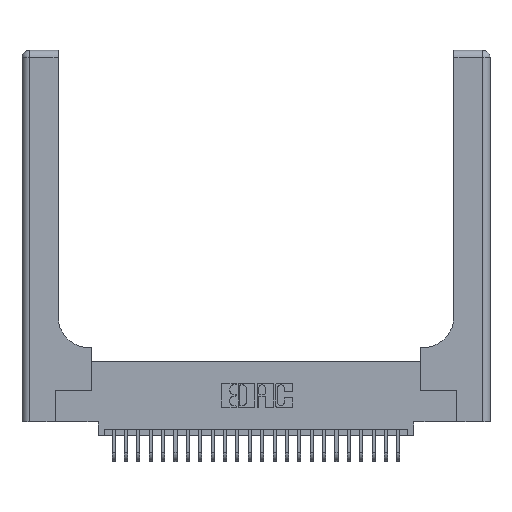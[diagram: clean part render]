
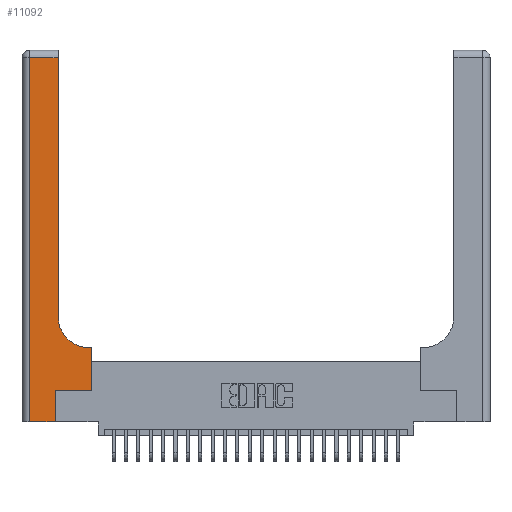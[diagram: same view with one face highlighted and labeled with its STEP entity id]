
A CAD part, top view. The second image highlights one B-rep face of the part: STEP entity #11092.
In plain terms, the highlighted planar face has unit normal (0, 0, 1).
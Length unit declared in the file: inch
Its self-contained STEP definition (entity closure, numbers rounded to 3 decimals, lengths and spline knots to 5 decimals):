
#36 = ORIENTED_EDGE ( 'NONE', *, *, #11155, .T. ) ;
#341 = VECTOR ( 'NONE', #14687, 39.37008 ) ;
#503 = CIRCLE ( 'NONE', #4987, 0.25 ) ;
#519 = EDGE_CURVE ( 'NONE', #6379, #22907, #762, .T. ) ;
#762 = LINE ( 'NONE', #20495, #17562 ) ;
#1103 = DIRECTION ( 'NONE',  ( -1., 0., 0. ) ) ;
#1154 = LINE ( 'NONE', #1720, #12187 ) ;
#1498 = DIRECTION ( 'NONE',  ( -1., 0., 0. ) ) ;
#1720 = CARTESIAN_POINT ( 'NONE',  ( 0.06, 3., 0.37 ) ) ;
#2502 = CARTESIAN_POINT ( 'NONE',  ( 0.5585, 0.6, 0.37 ) ) ;
#2640 = VECTOR ( 'NONE', #1103, 39.37008 ) ;
#2764 = EDGE_CURVE ( 'NONE', #15583, #7799, #26579, .T. ) ;
#2782 = DIRECTION ( 'NONE',  ( 0., 1., 0. ) ) ;
#3078 = AXIS2_PLACEMENT_3D ( 'NONE', #10267, #12429, #27551 ) ;
#3221 = CARTESIAN_POINT ( 'NONE',  ( 0.5585, 0.25, 0.37 ) ) ;
#4987 = AXIS2_PLACEMENT_3D ( 'NONE', #8377, #23534, #10559 ) ;
#5872 = PLANE ( 'NONE',  #3078 ) ;
#6274 = ORIENTED_EDGE ( 'NONE', *, *, #27512, .T. ) ;
#6373 = VERTEX_POINT ( 'NONE', #14166 ) ;
#6379 = VERTEX_POINT ( 'NONE', #25073 ) ;
#6664 = ORIENTED_EDGE ( 'NONE', *, *, #9556, .T. ) ;
#7328 = ORIENTED_EDGE ( 'NONE', *, *, #2764, .T. ) ;
#7674 = LINE ( 'NONE', #18972, #341 ) ;
#7799 = VERTEX_POINT ( 'NONE', #27784 ) ;
#8000 = CARTESIAN_POINT ( 'NONE',  ( 0.2915, 0.6, 0.37 ) ) ;
#8377 = CARTESIAN_POINT ( 'NONE',  ( 0.5415, 0.85, 0.37 ) ) ;
#9218 = LINE ( 'NONE', #12085, #2640 ) ;
#9556 = EDGE_CURVE ( 'NONE', #22907, #15828, #22045, .T. ) ;
#10267 = CARTESIAN_POINT ( 'NONE',  ( 0., 3., 0.37 ) ) ;
#10503 = VECTOR ( 'NONE', #2782, 39.37008 ) ;
#10559 = DIRECTION ( 'NONE',  ( 1., 0., 0. ) ) ;
#11092 = ADVANCED_FACE ( 'NONE', ( #12770 ), #5872, .F. ) ;
#11103 = VECTOR ( 'NONE', #18476, 39.37008 ) ;
#11155 = EDGE_CURVE ( 'NONE', #15828, #16306, #7674, .T. ) ;
#11172 = VECTOR ( 'NONE', #16464, 39.37008 ) ;
#12078 = ORIENTED_EDGE ( 'NONE', *, *, #519, .T. ) ;
#12085 = CARTESIAN_POINT ( 'NONE',  ( 0., 2.94, 0.37 ) ) ;
#12187 = VECTOR ( 'NONE', #14823, 39.37008 ) ;
#12429 = DIRECTION ( 'NONE',  ( 0., 0., -1. ) ) ;
#12770 = FACE_OUTER_BOUND ( 'NONE', #14096, .T. ) ;
#13562 = ORIENTED_EDGE ( 'NONE', *, *, #23172, .T. ) ;
#14096 = EDGE_LOOP ( 'NONE', ( #16411, #23236, #21832, #12078, #6664, #36, #6274, #7328, #13562 ) ) ;
#14166 = CARTESIAN_POINT ( 'NONE',  ( 0.06, 2.94, 0.37 ) ) ;
#14329 = VERTEX_POINT ( 'NONE', #17760 ) ;
#14687 = DIRECTION ( 'NONE',  ( 1., 0., 0. ) ) ;
#14823 = DIRECTION ( 'NONE',  ( 0., -1., 0. ) ) ;
#15583 = VERTEX_POINT ( 'NONE', #2502 ) ;
#15803 = EDGE_CURVE ( 'NONE', #14329, #6373, #9218, .T. ) ;
#15828 = VERTEX_POINT ( 'NONE', #27293 ) ;
#16306 = VERTEX_POINT ( 'NONE', #18227 ) ;
#16411 = ORIENTED_EDGE ( 'NONE', *, *, #26341, .T. ) ;
#16464 = DIRECTION ( 'NONE',  ( 0., 1., 0. ) ) ;
#16837 = EDGE_CURVE ( 'NONE', #6373, #6379, #1154, .T. ) ;
#17536 = LINE ( 'NONE', #3221, #11103 ) ;
#17562 = VECTOR ( 'NONE', #20458, 39.37008 ) ;
#17760 = CARTESIAN_POINT ( 'NONE',  ( 0.2915, 2.94, 0.37 ) ) ;
#18227 = CARTESIAN_POINT ( 'NONE',  ( 0.5585, 0.25, 0.37 ) ) ;
#18476 = DIRECTION ( 'NONE',  ( 0., 1., 0. ) ) ;
#18815 = CARTESIAN_POINT ( 'NONE',  ( 0.2915, 3., 0.37 ) ) ;
#18972 = CARTESIAN_POINT ( 'NONE',  ( 0.269, 0.25, 0.37 ) ) ;
#20424 = CARTESIAN_POINT ( 'NONE',  ( 0.269, 0., 0.37 ) ) ;
#20458 = DIRECTION ( 'NONE',  ( 1., 0., 0. ) ) ;
#20495 = CARTESIAN_POINT ( 'NONE',  ( 0., 0., 0.37 ) ) ;
#20854 = VECTOR ( 'NONE', #1498, 39.37008 ) ;
#21832 = ORIENTED_EDGE ( 'NONE', *, *, #16837, .T. ) ;
#22045 = LINE ( 'NONE', #26746, #10503 ) ;
#22907 = VERTEX_POINT ( 'NONE', #20424 ) ;
#23172 = EDGE_CURVE ( 'NONE', #7799, #27740, #503, .T. ) ;
#23236 = ORIENTED_EDGE ( 'NONE', *, *, #15803, .T. ) ;
#23488 = CARTESIAN_POINT ( 'NONE',  ( 0.2915, 0.85, 0.37 ) ) ;
#23534 = DIRECTION ( 'NONE',  ( 0., 0., -1. ) ) ;
#25073 = CARTESIAN_POINT ( 'NONE',  ( 0.06, 0., 0.37 ) ) ;
#26341 = EDGE_CURVE ( 'NONE', #27740, #14329, #27731, .T. ) ;
#26579 = LINE ( 'NONE', #8000, #20854 ) ;
#26746 = CARTESIAN_POINT ( 'NONE',  ( 0.269, 0., 0.37 ) ) ;
#27293 = CARTESIAN_POINT ( 'NONE',  ( 0.269, 0.25, 0.37 ) ) ;
#27512 = EDGE_CURVE ( 'NONE', #16306, #15583, #17536, .T. ) ;
#27551 = DIRECTION ( 'NONE',  ( -1., 0., 0. ) ) ;
#27731 = LINE ( 'NONE', #18815, #11172 ) ;
#27740 = VERTEX_POINT ( 'NONE', #23488 ) ;
#27784 = CARTESIAN_POINT ( 'NONE',  ( 0.5415, 0.6, 0.37 ) ) ;
